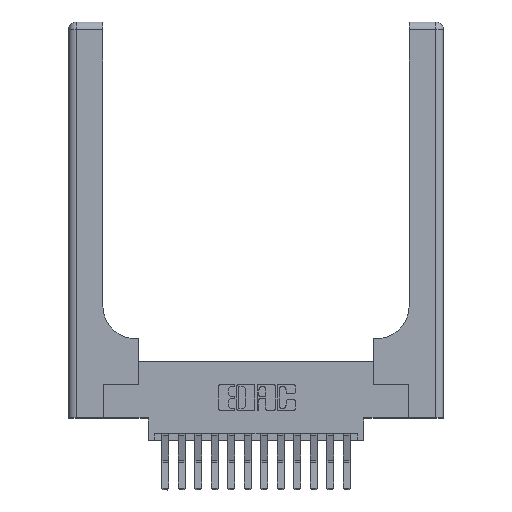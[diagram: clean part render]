
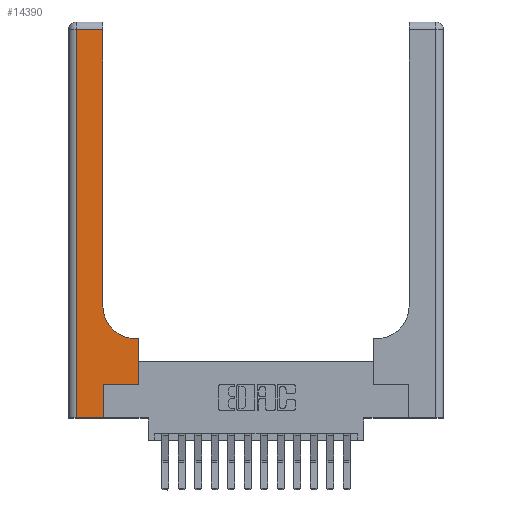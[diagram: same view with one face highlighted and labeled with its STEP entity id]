
A CAD part, top view. The second image highlights one B-rep face of the part: STEP entity #14390.
In plain terms, the highlighted planar face has unit normal (0, 0, 1).
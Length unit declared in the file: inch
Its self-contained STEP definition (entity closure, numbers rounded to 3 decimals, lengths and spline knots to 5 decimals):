
#816 = LINE ( 'NONE', #11874, #4010 ) ;
#1134 = DIRECTION ( 'NONE',  ( 1., 0., 0. ) ) ;
#1203 = CIRCLE ( 'NONE', #8371, 0.25 ) ;
#1583 = DIRECTION ( 'NONE',  ( 0., 0., -1. ) ) ;
#1710 = CARTESIAN_POINT ( 'NONE',  ( 0.51, 0.6, 0.37 ) ) ;
#1780 = DIRECTION ( 'NONE',  ( 1., 0., 0. ) ) ;
#2034 = VECTOR ( 'NONE', #11798, 39.37008 ) ;
#2881 = VECTOR ( 'NONE', #5581, 39.37008 ) ;
#2898 = CARTESIAN_POINT ( 'NONE',  ( 0.528, 0.25, 0.37 ) ) ;
#3002 = DIRECTION ( 'NONE',  ( -1., 0., 0. ) ) ;
#3186 = ORIENTED_EDGE ( 'NONE', *, *, #13814, .T. ) ;
#3219 = CARTESIAN_POINT ( 'NONE',  ( 0.06, 0., 0.37 ) ) ;
#3423 = ORIENTED_EDGE ( 'NONE', *, *, #8493, .T. ) ;
#3794 = FACE_OUTER_BOUND ( 'NONE', #4242, .T. ) ;
#3919 = DIRECTION ( 'NONE',  ( -1., 0., 0. ) ) ;
#4010 = VECTOR ( 'NONE', #9329, 39.37008 ) ;
#4069 = EDGE_CURVE ( 'NONE', #17039, #17271, #11765, .T. ) ;
#4242 = EDGE_LOOP ( 'NONE', ( #13355, #5815, #8565, #9284, #3186, #11785, #3423, #12846, #13285 ) ) ;
#5336 = VERTEX_POINT ( 'NONE', #1710 ) ;
#5581 = DIRECTION ( 'NONE',  ( 0., 1., 0. ) ) ;
#5727 = LINE ( 'NONE', #14981, #9674 ) ;
#5815 = ORIENTED_EDGE ( 'NONE', *, *, #13961, .T. ) ;
#6483 = LINE ( 'NONE', #14836, #2881 ) ;
#7152 = CARTESIAN_POINT ( 'NONE',  ( 0.26, 0.85, 0.37 ) ) ;
#7428 = VERTEX_POINT ( 'NONE', #14181 ) ;
#7937 = PLANE ( 'NONE',  #11787 ) ;
#8124 = DIRECTION ( 'NONE',  ( 0., -1., 0. ) ) ;
#8308 = VECTOR ( 'NONE', #15269, 39.37008 ) ;
#8371 = AXIS2_PLACEMENT_3D ( 'NONE', #9621, #1583, #10950 ) ;
#8492 = CARTESIAN_POINT ( 'NONE',  ( 0.265, 0.25, 0.37 ) ) ;
#8493 = EDGE_CURVE ( 'NONE', #15973, #10717, #6483, .T. ) ;
#8565 = ORIENTED_EDGE ( 'NONE', *, *, #4069, .T. ) ;
#8594 = VERTEX_POINT ( 'NONE', #7152 ) ;
#9055 = LINE ( 'NONE', #8492, #9474 ) ;
#9284 = ORIENTED_EDGE ( 'NONE', *, *, #16998, .T. ) ;
#9329 = DIRECTION ( 'NONE',  ( 0., 1., 0. ) ) ;
#9474 = VECTOR ( 'NONE', #1780, 39.37008 ) ;
#9621 = CARTESIAN_POINT ( 'NONE',  ( 0.51, 0.85, 0.37 ) ) ;
#9674 = VECTOR ( 'NONE', #3002, 39.37008 ) ;
#10512 = CARTESIAN_POINT ( 'NONE',  ( 0.265, 0.25, 0.37 ) ) ;
#10515 = CARTESIAN_POINT ( 'NONE',  ( 0., 3., 0.37 ) ) ;
#10568 = CARTESIAN_POINT ( 'NONE',  ( 0.06, 2.94, 0.37 ) ) ;
#10717 = VERTEX_POINT ( 'NONE', #12588 ) ;
#10950 = DIRECTION ( 'NONE',  ( 1., 0., 0. ) ) ;
#11175 = EDGE_CURVE ( 'NONE', #10717, #5336, #12243, .T. ) ;
#11442 = VECTOR ( 'NONE', #1134, 39.37008 ) ;
#11765 = LINE ( 'NONE', #16038, #15699 ) ;
#11785 = ORIENTED_EDGE ( 'NONE', *, *, #13001, .T. ) ;
#11787 = AXIS2_PLACEMENT_3D ( 'NONE', #10515, #11915, #3919 ) ;
#11798 = DIRECTION ( 'NONE',  ( 0., 1., 0. ) ) ;
#11874 = CARTESIAN_POINT ( 'NONE',  ( 0.265, 0., 0.37 ) ) ;
#11915 = DIRECTION ( 'NONE',  ( 0., 0., -1. ) ) ;
#12243 = LINE ( 'NONE', #12637, #8308 ) ;
#12588 = CARTESIAN_POINT ( 'NONE',  ( 0.528, 0.6, 0.37 ) ) ;
#12637 = CARTESIAN_POINT ( 'NONE',  ( 0.26, 0.6, 0.37 ) ) ;
#12705 = LINE ( 'NONE', #14397, #2034 ) ;
#12767 = VERTEX_POINT ( 'NONE', #10512 ) ;
#12846 = ORIENTED_EDGE ( 'NONE', *, *, #11175, .T. ) ;
#13001 = EDGE_CURVE ( 'NONE', #12767, #15973, #9055, .T. ) ;
#13285 = ORIENTED_EDGE ( 'NONE', *, *, #15987, .T. ) ;
#13355 = ORIENTED_EDGE ( 'NONE', *, *, #16975, .T. ) ;
#13814 = EDGE_CURVE ( 'NONE', #7428, #12767, #816, .T. ) ;
#13961 = EDGE_CURVE ( 'NONE', #15088, #17039, #5727, .T. ) ;
#14181 = CARTESIAN_POINT ( 'NONE',  ( 0.265, 0., 0.37 ) ) ;
#14390 = ADVANCED_FACE ( 'NONE', ( #3794 ), #7937, .F. ) ;
#14397 = CARTESIAN_POINT ( 'NONE',  ( 0.26, 3., 0.37 ) ) ;
#14455 = CARTESIAN_POINT ( 'NONE',  ( 0., 0., 0.37 ) ) ;
#14836 = CARTESIAN_POINT ( 'NONE',  ( 0.528, 0.25, 0.37 ) ) ;
#14948 = LINE ( 'NONE', #14455, #11442 ) ;
#14981 = CARTESIAN_POINT ( 'NONE',  ( 0., 2.94, 0.37 ) ) ;
#15088 = VERTEX_POINT ( 'NONE', #17015 ) ;
#15269 = DIRECTION ( 'NONE',  ( -1., 0., 0. ) ) ;
#15699 = VECTOR ( 'NONE', #8124, 39.37008 ) ;
#15973 = VERTEX_POINT ( 'NONE', #2898 ) ;
#15987 = EDGE_CURVE ( 'NONE', #5336, #8594, #1203, .T. ) ;
#16038 = CARTESIAN_POINT ( 'NONE',  ( 0.06, 3., 0.37 ) ) ;
#16975 = EDGE_CURVE ( 'NONE', #8594, #15088, #12705, .T. ) ;
#16998 = EDGE_CURVE ( 'NONE', #17271, #7428, #14948, .T. ) ;
#17015 = CARTESIAN_POINT ( 'NONE',  ( 0.26, 2.94, 0.37 ) ) ;
#17039 = VERTEX_POINT ( 'NONE', #10568 ) ;
#17271 = VERTEX_POINT ( 'NONE', #3219 ) ;
